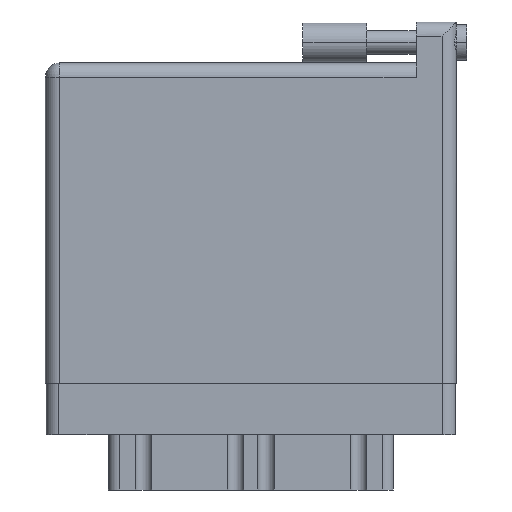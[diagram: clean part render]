
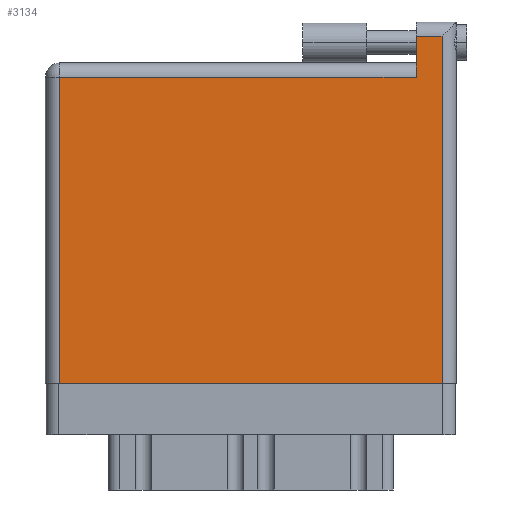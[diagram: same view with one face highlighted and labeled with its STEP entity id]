
A CAD part, front view. The second image highlights one B-rep face of the part: STEP entity #3134.
In plain terms, the highlighted face is planar.
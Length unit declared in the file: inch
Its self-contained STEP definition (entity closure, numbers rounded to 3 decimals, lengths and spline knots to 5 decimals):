
#267 = VERTEX_POINT ( 'NONE', #25765 ) ;
#1928 = VECTOR ( 'NONE', #26284, 39.37008 ) ;
#3100 = ORIENTED_EDGE ( 'NONE', *, *, #23609, .T. ) ;
#3134 = ADVANCED_FACE ( 'NONE', ( #19861 ), #5804, .F. ) ;
#3194 = DIRECTION ( 'NONE',  ( -1., 0., 0. ) ) ;
#3460 = ORIENTED_EDGE ( 'NONE', *, *, #16041, .T. ) ;
#3904 = DIRECTION ( 'NONE',  ( 1., 0., 0. ) ) ;
#4563 = CARTESIAN_POINT ( 'NONE',  ( 0., 1.696, 0. ) ) ;
#5004 = ORIENTED_EDGE ( 'NONE', *, *, #30668, .T. ) ;
#5804 = PLANE ( 'NONE',  #33954 ) ;
#6528 = EDGE_CURVE ( 'NONE', #267, #7578, #6647, .T. ) ;
#6647 = LINE ( 'NONE', #22303, #27300 ) ;
#7578 = VERTEX_POINT ( 'NONE', #11519 ) ;
#7907 = VERTEX_POINT ( 'NONE', #31208 ) ;
#9121 = CARTESIAN_POINT ( 'NONE',  ( 0., 0., 0. ) ) ;
#9296 = CARTESIAN_POINT ( 'NONE',  ( 1.938, 0., 0. ) ) ;
#9456 = LINE ( 'NONE', #9121, #16917 ) ;
#11519 = CARTESIAN_POINT ( 'NONE',  ( 0.07, 1.496, 0. ) ) ;
#12518 = VECTOR ( 'NONE', #15194, 39.37008 ) ;
#13864 = EDGE_CURVE ( 'NONE', #22693, #17597, #9456, .T. ) ;
#14472 = ORIENTED_EDGE ( 'NONE', *, *, #6528, .T. ) ;
#14832 = DIRECTION ( 'NONE',  ( -1., 0., 0. ) ) ;
#15054 = ORIENTED_EDGE ( 'NONE', *, *, #33242, .T. ) ;
#15194 = DIRECTION ( 'NONE',  ( -1., 0., 0. ) ) ;
#16041 = EDGE_CURVE ( 'NONE', #17597, #33117, #31359, .T. ) ;
#16425 = CARTESIAN_POINT ( 'NONE',  ( 0., 1.566, 0. ) ) ;
#16917 = VECTOR ( 'NONE', #3904, 39.37008 ) ;
#17274 = CARTESIAN_POINT ( 'NONE',  ( 1.938, 1.696, 0. ) ) ;
#17349 = CARTESIAN_POINT ( 'NONE',  ( 0.07, 0., 0. ) ) ;
#17582 = CARTESIAN_POINT ( 'NONE',  ( 1.938, 1.766, 0. ) ) ;
#17597 = VERTEX_POINT ( 'NONE', #9296 ) ;
#19612 = CARTESIAN_POINT ( 'NONE',  ( 1.811, 1.766, 0. ) ) ;
#19861 = FACE_OUTER_BOUND ( 'NONE', #33582, .T. ) ;
#21215 = ORIENTED_EDGE ( 'NONE', *, *, #13864, .T. ) ;
#22303 = CARTESIAN_POINT ( 'NONE',  ( 0., 1.496, 0. ) ) ;
#22409 = LINE ( 'NONE', #19612, #31319 ) ;
#22693 = VERTEX_POINT ( 'NONE', #17349 ) ;
#23609 = EDGE_CURVE ( 'NONE', #7578, #22693, #32817, .T. ) ;
#24871 = DIRECTION ( 'NONE',  ( 0., -1., 0. ) ) ;
#25765 = CARTESIAN_POINT ( 'NONE',  ( 1.811, 1.496, 0. ) ) ;
#26284 = DIRECTION ( 'NONE',  ( 0., 1., 0. ) ) ;
#27062 = DIRECTION ( 'NONE',  ( 0., 0., -1. ) ) ;
#27073 = DIRECTION ( 'NONE',  ( 0., -1., 0. ) ) ;
#27300 = VECTOR ( 'NONE', #14832, 39.37008 ) ;
#28439 = LINE ( 'NONE', #4563, #12518 ) ;
#29825 = VECTOR ( 'NONE', #27073, 39.37008 ) ;
#30668 = EDGE_CURVE ( 'NONE', #7907, #267, #22409, .T. ) ;
#31208 = CARTESIAN_POINT ( 'NONE',  ( 1.811, 1.696, 0. ) ) ;
#31319 = VECTOR ( 'NONE', #24871, 39.37008 ) ;
#31359 = LINE ( 'NONE', #17582, #1928 ) ;
#32817 = LINE ( 'NONE', #33445, #29825 ) ;
#33117 = VERTEX_POINT ( 'NONE', #17274 ) ;
#33242 = EDGE_CURVE ( 'NONE', #33117, #7907, #28439, .T. ) ;
#33445 = CARTESIAN_POINT ( 'NONE',  ( 0.07, 0., 0. ) ) ;
#33582 = EDGE_LOOP ( 'NONE', ( #21215, #3460, #15054, #5004, #14472, #3100 ) ) ;
#33954 = AXIS2_PLACEMENT_3D ( 'NONE', #16425, #27062, #3194 ) ;
